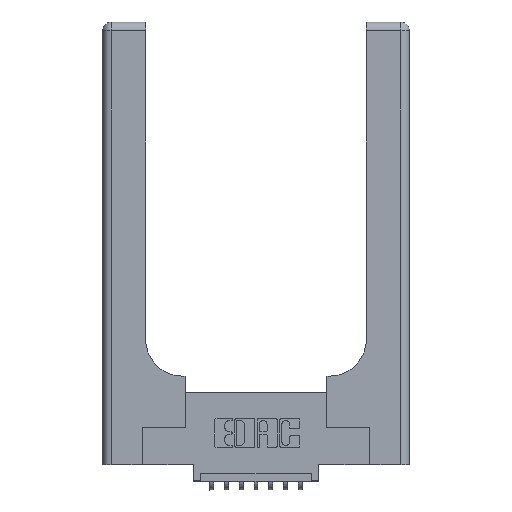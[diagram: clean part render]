
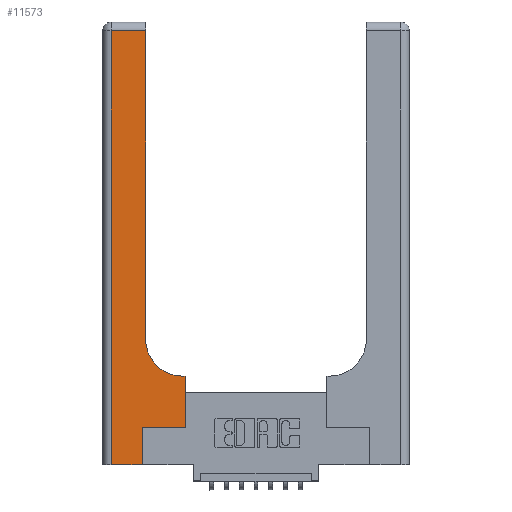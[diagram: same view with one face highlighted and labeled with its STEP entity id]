
A CAD part, top view. The second image highlights one B-rep face of the part: STEP entity #11573.
In plain terms, the highlighted planar face has unit normal (0, 0, 1).
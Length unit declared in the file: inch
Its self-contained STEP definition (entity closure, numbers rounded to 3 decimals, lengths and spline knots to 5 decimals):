
#18 = CARTESIAN_POINT ( 'NONE',  ( 0.5415, 0.6, 0.37 ) ) ;
#155 = ORIENTED_EDGE ( 'NONE', *, *, #8360, .T. ) ;
#577 = EDGE_CURVE ( 'NONE', #13357, #6131, #7073, .T. ) ;
#714 = VECTOR ( 'NONE', #7737, 39.37008 ) ;
#1145 = CARTESIAN_POINT ( 'NONE',  ( 0., 2.94, 0.37 ) ) ;
#1182 = VECTOR ( 'NONE', #14210, 39.37008 ) ;
#1264 = EDGE_CURVE ( 'NONE', #4418, #4833, #12808, .T. ) ;
#1481 = VERTEX_POINT ( 'NONE', #1492 ) ;
#1492 = CARTESIAN_POINT ( 'NONE',  ( 0.06, 2.94, 0.37 ) ) ;
#1663 = LINE ( 'NONE', #11787, #10051 ) ;
#2384 = AXIS2_PLACEMENT_3D ( 'NONE', #8929, #8874, #12457 ) ;
#2865 = FACE_OUTER_BOUND ( 'NONE', #9067, .T. ) ;
#2901 = VECTOR ( 'NONE', #7561, 39.37008 ) ;
#2926 = DIRECTION ( 'NONE',  ( 1., 0., 0. ) ) ;
#3280 = ORIENTED_EDGE ( 'NONE', *, *, #5163, .T. ) ;
#3338 = VECTOR ( 'NONE', #2926, 39.37008 ) ;
#3458 = EDGE_CURVE ( 'NONE', #7949, #11947, #3648, .T. ) ;
#3648 = LINE ( 'NONE', #10168, #2901 ) ;
#3872 = LINE ( 'NONE', #13594, #714 ) ;
#4000 = DIRECTION ( 'NONE',  ( 0., 0., -1. ) ) ;
#4167 = VERTEX_POINT ( 'NONE', #18 ) ;
#4225 = CARTESIAN_POINT ( 'NONE',  ( 0., 3., 0.37 ) ) ;
#4418 = VERTEX_POINT ( 'NONE', #14160 ) ;
#4452 = EDGE_CURVE ( 'NONE', #11947, #1481, #12343, .T. ) ;
#4584 = CARTESIAN_POINT ( 'NONE',  ( 0.269, 0., 0.37 ) ) ;
#4743 = VECTOR ( 'NONE', #6136, 39.37008 ) ;
#4833 = VERTEX_POINT ( 'NONE', #8028 ) ;
#5163 = EDGE_CURVE ( 'NONE', #1481, #13357, #13090, .T. ) ;
#5345 = ORIENTED_EDGE ( 'NONE', *, *, #4452, .T. ) ;
#5375 = DIRECTION ( 'NONE',  ( -1., 0., 0. ) ) ;
#5893 = DIRECTION ( 'NONE',  ( 1., 0., 0. ) ) ;
#5978 = EDGE_CURVE ( 'NONE', #4167, #7949, #6381, .T. ) ;
#6131 = VERTEX_POINT ( 'NONE', #4584 ) ;
#6136 = DIRECTION ( 'NONE',  ( 0., -1., 0. ) ) ;
#6345 = CARTESIAN_POINT ( 'NONE',  ( 0.06, 0., 0.37 ) ) ;
#6381 = CIRCLE ( 'NONE', #2384, 0.25 ) ;
#6419 = CARTESIAN_POINT ( 'NONE',  ( 0.269, 0.25, 0.37 ) ) ;
#6501 = CARTESIAN_POINT ( 'NONE',  ( 0.269, 0.25, 0.37 ) ) ;
#7073 = LINE ( 'NONE', #11803, #8019 ) ;
#7092 = ORIENTED_EDGE ( 'NONE', *, *, #577, .T. ) ;
#7437 = ORIENTED_EDGE ( 'NONE', *, *, #1264, .T. ) ;
#7438 = EDGE_CURVE ( 'NONE', #4833, #4167, #1663, .T. ) ;
#7561 = DIRECTION ( 'NONE',  ( 0., 1., 0. ) ) ;
#7737 = DIRECTION ( 'NONE',  ( 0., 1., 0. ) ) ;
#7928 = ORIENTED_EDGE ( 'NONE', *, *, #5978, .T. ) ;
#7949 = VERTEX_POINT ( 'NONE', #8203 ) ;
#8019 = VECTOR ( 'NONE', #5893, 39.37008 ) ;
#8028 = CARTESIAN_POINT ( 'NONE',  ( 0.5585, 0.6, 0.37 ) ) ;
#8203 = CARTESIAN_POINT ( 'NONE',  ( 0.2915, 0.85, 0.37 ) ) ;
#8360 = EDGE_CURVE ( 'NONE', #6131, #9404, #3872, .T. ) ;
#8859 = EDGE_CURVE ( 'NONE', #9404, #4418, #9486, .T. ) ;
#8874 = DIRECTION ( 'NONE',  ( 0., 0., -1. ) ) ;
#8929 = CARTESIAN_POINT ( 'NONE',  ( 0.5415, 0.85, 0.37 ) ) ;
#9067 = EDGE_LOOP ( 'NONE', ( #9462, #5345, #3280, #7092, #155, #10350, #7437, #9133, #7928 ) ) ;
#9133 = ORIENTED_EDGE ( 'NONE', *, *, #7438, .T. ) ;
#9404 = VERTEX_POINT ( 'NONE', #6501 ) ;
#9462 = ORIENTED_EDGE ( 'NONE', *, *, #3458, .T. ) ;
#9486 = LINE ( 'NONE', #6419, #3338 ) ;
#10051 = VECTOR ( 'NONE', #14132, 39.37008 ) ;
#10168 = CARTESIAN_POINT ( 'NONE',  ( 0.2915, 3., 0.37 ) ) ;
#10350 = ORIENTED_EDGE ( 'NONE', *, *, #8859, .T. ) ;
#10710 = AXIS2_PLACEMENT_3D ( 'NONE', #4225, #4000, #5375 ) ;
#11573 = ADVANCED_FACE ( 'NONE', ( #2865 ), #13684, .F. ) ;
#11787 = CARTESIAN_POINT ( 'NONE',  ( 0.2915, 0.6, 0.37 ) ) ;
#11803 = CARTESIAN_POINT ( 'NONE',  ( 0., 0., 0.37 ) ) ;
#11947 = VERTEX_POINT ( 'NONE', #15303 ) ;
#12343 = LINE ( 'NONE', #1145, #1182 ) ;
#12457 = DIRECTION ( 'NONE',  ( 1., 0., 0. ) ) ;
#12808 = LINE ( 'NONE', #14604, #13368 ) ;
#13090 = LINE ( 'NONE', #14512, #4743 ) ;
#13357 = VERTEX_POINT ( 'NONE', #6345 ) ;
#13368 = VECTOR ( 'NONE', #13967, 39.37008 ) ;
#13594 = CARTESIAN_POINT ( 'NONE',  ( 0.269, 0., 0.37 ) ) ;
#13684 = PLANE ( 'NONE',  #10710 ) ;
#13967 = DIRECTION ( 'NONE',  ( 0., 1., 0. ) ) ;
#14132 = DIRECTION ( 'NONE',  ( -1., 0., 0. ) ) ;
#14160 = CARTESIAN_POINT ( 'NONE',  ( 0.5585, 0.25, 0.37 ) ) ;
#14210 = DIRECTION ( 'NONE',  ( -1., 0., 0. ) ) ;
#14512 = CARTESIAN_POINT ( 'NONE',  ( 0.06, 3., 0.37 ) ) ;
#14604 = CARTESIAN_POINT ( 'NONE',  ( 0.5585, 0.25, 0.37 ) ) ;
#15303 = CARTESIAN_POINT ( 'NONE',  ( 0.2915, 2.94, 0.37 ) ) ;
